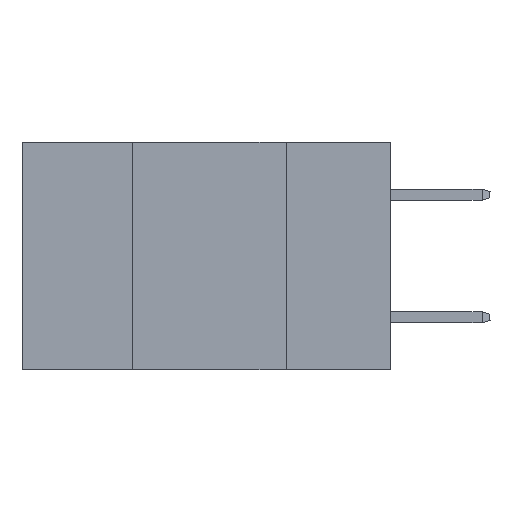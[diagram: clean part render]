
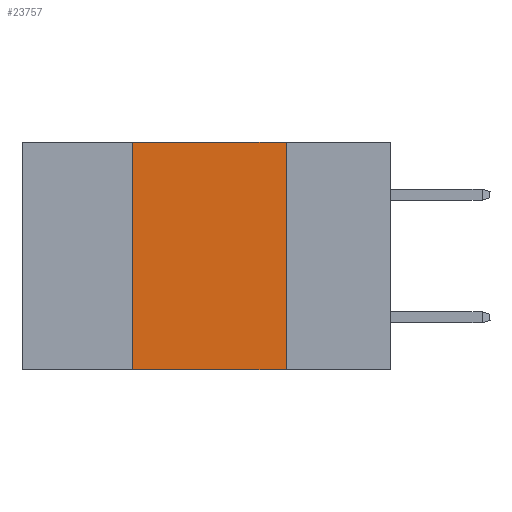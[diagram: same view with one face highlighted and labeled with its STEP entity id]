
A CAD part, left-side view. The second image highlights one B-rep face of the part: STEP entity #23757.
In plain terms, the highlighted planar face has unit normal (-1, 0, 0).
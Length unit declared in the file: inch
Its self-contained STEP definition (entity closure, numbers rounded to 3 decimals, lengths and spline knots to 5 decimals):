
#68 = CARTESIAN_POINT ( 'NONE',  ( 0., 0.6, 0. ) ) ;
#477 = ORIENTED_EDGE ( 'NONE', *, *, #7270, .F. ) ;
#1203 = ORIENTED_EDGE ( 'NONE', *, *, #25103, .F. ) ;
#1323 = DIRECTION ( 'NONE',  ( 1., 0., 0. ) ) ;
#4601 = DIRECTION ( 'NONE',  ( 0., -1., 0. ) ) ;
#4853 = EDGE_LOOP ( 'NONE', ( #23108, #477, #1203, #26616 ) ) ;
#5282 = FACE_OUTER_BOUND ( 'NONE', #4853, .T. ) ;
#5474 = EDGE_CURVE ( 'NONE', #28110, #11903, #11767, .T. ) ;
#6131 = CARTESIAN_POINT ( 'NONE',  ( 0., 0.42, -0.37 ) ) ;
#7193 = CARTESIAN_POINT ( 'NONE',  ( 0., 0.6, -0.37 ) ) ;
#7270 = EDGE_CURVE ( 'NONE', #17977, #28750, #10208, .T. ) ;
#8151 = CARTESIAN_POINT ( 'NONE',  ( 0., 0.42, 0. ) ) ;
#10208 = LINE ( 'NONE', #68, #21471 ) ;
#10343 = DIRECTION ( 'NONE',  ( 0., 0., -1. ) ) ;
#10486 = CARTESIAN_POINT ( 'NONE',  ( 0., 0.17, -0.37 ) ) ;
#11767 = LINE ( 'NONE', #7193, #17082 ) ;
#11903 = VERTEX_POINT ( 'NONE', #10486 ) ;
#12173 = CARTESIAN_POINT ( 'NONE',  ( 0., 0.42, 0. ) ) ;
#12481 = EDGE_CURVE ( 'NONE', #28750, #11903, #28797, .T. ) ;
#12619 = CARTESIAN_POINT ( 'NONE',  ( 0., 0.6, 0. ) ) ;
#17082 = VECTOR ( 'NONE', #27448, 39.37008 ) ;
#17188 = DIRECTION ( 'NONE',  ( 0., 0., -1. ) ) ;
#17254 = LINE ( 'NONE', #8151, #23876 ) ;
#17679 = VECTOR ( 'NONE', #10343, 39.37008 ) ;
#17977 = VERTEX_POINT ( 'NONE', #12173 ) ;
#21471 = VECTOR ( 'NONE', #4601, 39.37008 ) ;
#23108 = ORIENTED_EDGE ( 'NONE', *, *, #12481, .F. ) ;
#23757 = ADVANCED_FACE ( 'NONE', ( #5282 ), #26070, .F. ) ;
#23836 = CARTESIAN_POINT ( 'NONE',  ( 0., 0.17, 0. ) ) ;
#23876 = VECTOR ( 'NONE', #23935, 39.37008 ) ;
#23935 = DIRECTION ( 'NONE',  ( 0., 0., 1. ) ) ;
#25103 = EDGE_CURVE ( 'NONE', #28110, #17977, #17254, .T. ) ;
#26070 = PLANE ( 'NONE',  #26217 ) ;
#26175 = CARTESIAN_POINT ( 'NONE',  ( 0., 0.17, 0. ) ) ;
#26217 = AXIS2_PLACEMENT_3D ( 'NONE', #12619, #1323, #17188 ) ;
#26616 = ORIENTED_EDGE ( 'NONE', *, *, #5474, .T. ) ;
#27448 = DIRECTION ( 'NONE',  ( 0., -1., 0. ) ) ;
#28110 = VERTEX_POINT ( 'NONE', #6131 ) ;
#28750 = VERTEX_POINT ( 'NONE', #26175 ) ;
#28797 = LINE ( 'NONE', #23836, #17679 ) ;
